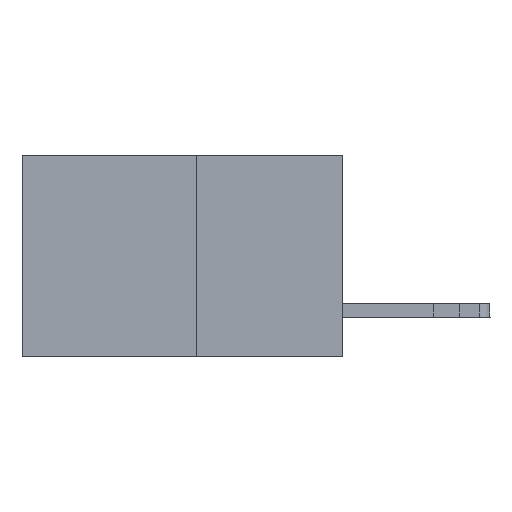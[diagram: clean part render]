
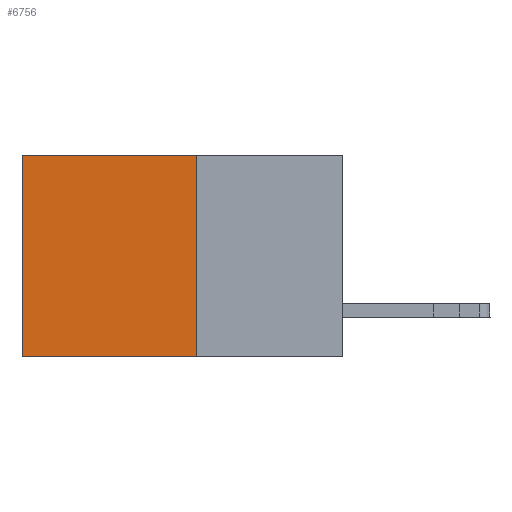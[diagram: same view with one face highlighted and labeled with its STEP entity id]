
A CAD part, left-side view. The second image highlights one B-rep face of the part: STEP entity #6756.
In plain terms, the highlighted planar face has unit normal (-1, 0, 0).
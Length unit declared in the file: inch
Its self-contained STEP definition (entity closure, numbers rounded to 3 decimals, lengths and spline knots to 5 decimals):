
#381 = PLANE ( 'NONE',  #8375 ) ;
#693 = EDGE_CURVE ( 'NONE', #8016, #12297, #18372, .T. ) ;
#781 = VECTOR ( 'NONE', #7182, 39.37008 ) ;
#2201 = VECTOR ( 'NONE', #8171, 39.37008 ) ;
#2367 = DIRECTION ( 'NONE',  ( 0., 0., -1. ) ) ;
#2506 = DIRECTION ( 'NONE',  ( 0., 0., -1. ) ) ;
#3335 = CARTESIAN_POINT ( 'NONE',  ( 0.277, 0.27, 0. ) ) ;
#4424 = CARTESIAN_POINT ( 'NONE',  ( 0.277, 0.27, 0. ) ) ;
#5760 = CARTESIAN_POINT ( 'NONE',  ( 0.277, 0.27, -0.37 ) ) ;
#5855 = CARTESIAN_POINT ( 'NONE',  ( 0.277, 0.59, -0.37 ) ) ;
#6756 = ADVANCED_FACE ( 'NONE', ( #18547 ), #381, .F. ) ;
#7182 = DIRECTION ( 'NONE',  ( 0., 1., 0. ) ) ;
#7766 = EDGE_CURVE ( 'NONE', #8016, #25627, #22936, .T. ) ;
#8016 = VERTEX_POINT ( 'NONE', #4424 ) ;
#8139 = ORIENTED_EDGE ( 'NONE', *, *, #18774, .T. ) ;
#8171 = DIRECTION ( 'NONE',  ( 0., 0., -1. ) ) ;
#8345 = CARTESIAN_POINT ( 'NONE',  ( 0.277, 0.27, -0.37 ) ) ;
#8375 = AXIS2_PLACEMENT_3D ( 'NONE', #8345, #10087, #2506 ) ;
#9079 = DIRECTION ( 'NONE',  ( 0., 1., 0. ) ) ;
#10087 = DIRECTION ( 'NONE',  ( 1., 0., 0. ) ) ;
#11742 = ORIENTED_EDGE ( 'NONE', *, *, #693, .F. ) ;
#12297 = VERTEX_POINT ( 'NONE', #5760 ) ;
#12984 = CARTESIAN_POINT ( 'NONE',  ( 0.277, 0.59, -0.37 ) ) ;
#13002 = ORIENTED_EDGE ( 'NONE', *, *, #7766, .T. ) ;
#13406 = EDGE_LOOP ( 'NONE', ( #8139, #25586, #11742, #13002 ) ) ;
#14029 = VERTEX_POINT ( 'NONE', #5855 ) ;
#17909 = VECTOR ( 'NONE', #2367, 39.37008 ) ;
#18372 = LINE ( 'NONE', #23819, #2201 ) ;
#18547 = FACE_OUTER_BOUND ( 'NONE', #13406, .T. ) ;
#18774 = EDGE_CURVE ( 'NONE', #25627, #14029, #20659, .T. ) ;
#18899 = VECTOR ( 'NONE', #9079, 39.37008 ) ;
#19075 = CARTESIAN_POINT ( 'NONE',  ( 0.277, 0.59, 0. ) ) ;
#19552 = LINE ( 'NONE', #25112, #18899 ) ;
#20659 = LINE ( 'NONE', #12984, #17909 ) ;
#22936 = LINE ( 'NONE', #3335, #781 ) ;
#23819 = CARTESIAN_POINT ( 'NONE',  ( 0.277, 0.27, -0.37 ) ) ;
#25112 = CARTESIAN_POINT ( 'NONE',  ( 0.277, 0.27, -0.37 ) ) ;
#25586 = ORIENTED_EDGE ( 'NONE', *, *, #26049, .F. ) ;
#25627 = VERTEX_POINT ( 'NONE', #19075 ) ;
#26049 = EDGE_CURVE ( 'NONE', #12297, #14029, #19552, .T. ) ;
